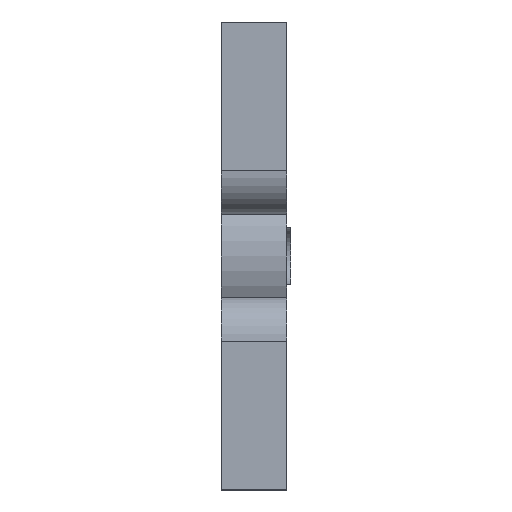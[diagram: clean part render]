
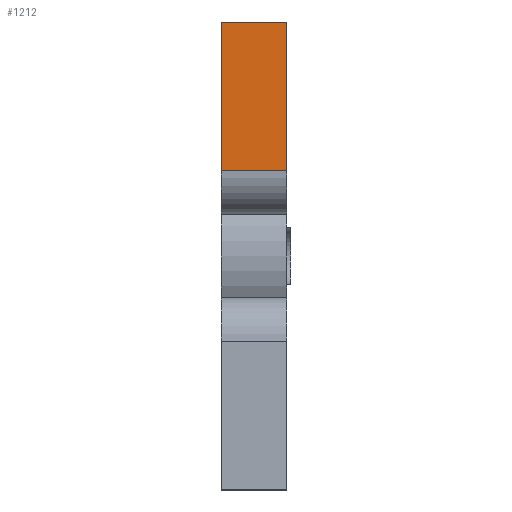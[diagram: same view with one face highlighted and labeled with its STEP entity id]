
A CAD part, left-side view. The second image highlights one B-rep face of the part: STEP entity #1212.
In plain terms, the highlighted planar face has unit normal (-1, 0, 0).
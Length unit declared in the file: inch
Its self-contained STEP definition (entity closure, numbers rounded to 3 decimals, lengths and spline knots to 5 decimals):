
#5 = VERTEX_POINT ( 'NONE', #1411 ) ;
#50 = LINE ( 'NONE', #1116, #474 ) ;
#82 = EDGE_LOOP ( 'NONE', ( #1273, #1406, #234, #757 ) ) ;
#234 = ORIENTED_EDGE ( 'NONE', *, *, #765, .T. ) ;
#264 = LINE ( 'NONE', #1657, #1137 ) ;
#295 = EDGE_CURVE ( 'NONE', #1210, #522, #264, .T. ) ;
#356 = VECTOR ( 'NONE', #1106, 39.37008 ) ;
#469 = EDGE_CURVE ( 'NONE', #1179, #5, #1049, .T. ) ;
#474 = VECTOR ( 'NONE', #1128, 39.37008 ) ;
#522 = VERTEX_POINT ( 'NONE', #1365 ) ;
#608 = AXIS2_PLACEMENT_3D ( 'NONE', #721, #715, #713 ) ;
#713 = DIRECTION ( 'NONE',  ( 0., 0., 1. ) ) ;
#715 = DIRECTION ( 'NONE',  ( -1., 0., 0. ) ) ;
#721 = CARTESIAN_POINT ( 'NONE',  ( 0.175, -0.71954, 0.6 ) ) ;
#733 = CARTESIAN_POINT ( 'NONE',  ( 0.175, 0.15, 0.26 ) ) ;
#736 = CARTESIAN_POINT ( 'NONE',  ( 0.175, 0.3, 0.26 ) ) ;
#757 = ORIENTED_EDGE ( 'NONE', *, *, #469, .F. ) ;
#761 = EDGE_CURVE ( 'NONE', #1210, #1179, #50, .T. ) ;
#763 = PLANE ( 'NONE',  #608 ) ;
#765 = EDGE_CURVE ( 'NONE', #522, #5, #866, .T. ) ;
#866 = LINE ( 'NONE', #1113, #356 ) ;
#1049 = LINE ( 'NONE', #1424, #1366 ) ;
#1106 = DIRECTION ( 'NONE',  ( 0., 1., 0. ) ) ;
#1113 = CARTESIAN_POINT ( 'NONE',  ( 0.175, -0.71954, 0.6 ) ) ;
#1116 = CARTESIAN_POINT ( 'NONE',  ( 0.175, -0.71954, 0.26 ) ) ;
#1128 = DIRECTION ( 'NONE',  ( 0., 1., 0. ) ) ;
#1137 = VECTOR ( 'NONE', #1655, 39.37008 ) ;
#1179 = VERTEX_POINT ( 'NONE', #736 ) ;
#1210 = VERTEX_POINT ( 'NONE', #733 ) ;
#1212 = ADVANCED_FACE ( 'NONE', ( #1704 ), #763, .T. ) ;
#1273 = ORIENTED_EDGE ( 'NONE', *, *, #761, .F. ) ;
#1365 = CARTESIAN_POINT ( 'NONE',  ( 0.175, 0.15, 0.6 ) ) ;
#1366 = VECTOR ( 'NONE', #1445, 39.37008 ) ;
#1406 = ORIENTED_EDGE ( 'NONE', *, *, #295, .T. ) ;
#1411 = CARTESIAN_POINT ( 'NONE',  ( 0.175, 0.3, 0.6 ) ) ;
#1424 = CARTESIAN_POINT ( 'NONE',  ( 0.175, 0.3, 0.6 ) ) ;
#1445 = DIRECTION ( 'NONE',  ( 0., 0., 1. ) ) ;
#1655 = DIRECTION ( 'NONE',  ( 0., 0., 1. ) ) ;
#1657 = CARTESIAN_POINT ( 'NONE',  ( 0.175, 0.15, 0.6 ) ) ;
#1704 = FACE_OUTER_BOUND ( 'NONE', #82, .T. ) ;
